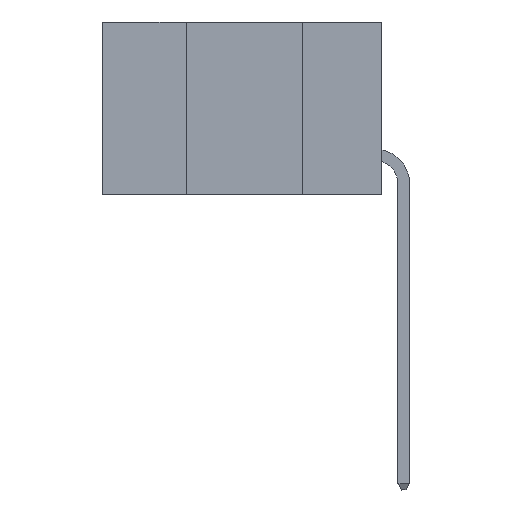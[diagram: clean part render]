
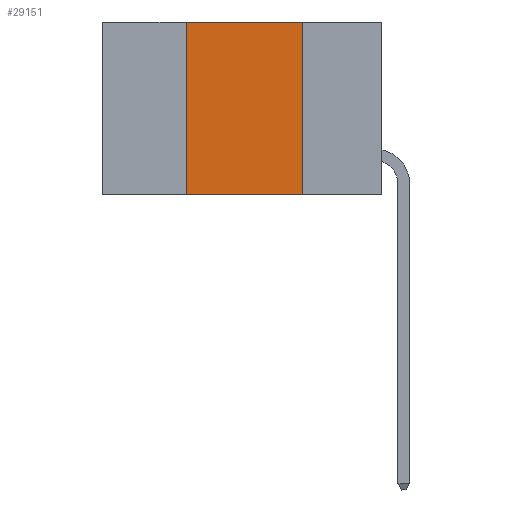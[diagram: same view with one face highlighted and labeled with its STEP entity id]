
A CAD part, left-side view. The second image highlights one B-rep face of the part: STEP entity #29151.
In plain terms, the highlighted planar face has unit normal (-1, 0, 0).
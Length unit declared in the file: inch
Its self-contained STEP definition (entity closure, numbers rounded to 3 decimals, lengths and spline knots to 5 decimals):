
#440 = ORIENTED_EDGE ( 'NONE', *, *, #24270, .F. ) ;
#1326 = CARTESIAN_POINT ( 'NONE',  ( 0., 0.17, 0. ) ) ;
#2971 = CARTESIAN_POINT ( 'NONE',  ( 0., 0.6, 0. ) ) ;
#3583 = VECTOR ( 'NONE', #29162, 39.37008 ) ;
#5345 = EDGE_CURVE ( 'NONE', #27842, #25203, #32969, .T. ) ;
#6522 = DIRECTION ( 'NONE',  ( 1., 0., 0. ) ) ;
#7519 = EDGE_CURVE ( 'NONE', #18928, #25203, #37913, .T. ) ;
#8083 = VECTOR ( 'NONE', #22757, 39.37008 ) ;
#9862 = CARTESIAN_POINT ( 'NONE',  ( 0., 0.42, -0.37 ) ) ;
#12090 = CARTESIAN_POINT ( 'NONE',  ( 0., 0.42, 0. ) ) ;
#13433 = CARTESIAN_POINT ( 'NONE',  ( 0., 0.6, 0. ) ) ;
#14147 = CARTESIAN_POINT ( 'NONE',  ( 0., 0.42, 0. ) ) ;
#14149 = DIRECTION ( 'NONE',  ( 0., 0., -1. ) ) ;
#16979 = CARTESIAN_POINT ( 'NONE',  ( 0., 0.17, 0. ) ) ;
#17227 = DIRECTION ( 'NONE',  ( 0., 0., -1. ) ) ;
#17507 = LINE ( 'NONE', #13433, #3583 ) ;
#18928 = VERTEX_POINT ( 'NONE', #9862 ) ;
#20367 = AXIS2_PLACEMENT_3D ( 'NONE', #2971, #6522, #14149 ) ;
#21437 = DIRECTION ( 'NONE',  ( 0., -1., 0. ) ) ;
#22757 = DIRECTION ( 'NONE',  ( 0., 0., 1. ) ) ;
#24270 = EDGE_CURVE ( 'NONE', #46572, #27842, #17507, .T. ) ;
#24780 = VECTOR ( 'NONE', #21437, 39.37008 ) ;
#25203 = VERTEX_POINT ( 'NONE', #30725 ) ;
#27842 = VERTEX_POINT ( 'NONE', #1326 ) ;
#29151 = ADVANCED_FACE ( 'NONE', ( #37261 ), #30114, .F. ) ;
#29162 = DIRECTION ( 'NONE',  ( 0., -1., 0. ) ) ;
#30036 = CARTESIAN_POINT ( 'NONE',  ( 0., 0.6, -0.37 ) ) ;
#30114 = PLANE ( 'NONE',  #20367 ) ;
#30371 = LINE ( 'NONE', #14147, #8083 ) ;
#30725 = CARTESIAN_POINT ( 'NONE',  ( 0., 0.17, -0.37 ) ) ;
#31342 = ORIENTED_EDGE ( 'NONE', *, *, #7519, .T. ) ;
#32969 = LINE ( 'NONE', #16979, #45984 ) ;
#37261 = FACE_OUTER_BOUND ( 'NONE', #41971, .T. ) ;
#37913 = LINE ( 'NONE', #30036, #24780 ) ;
#41512 = EDGE_CURVE ( 'NONE', #18928, #46572, #30371, .T. ) ;
#41971 = EDGE_LOOP ( 'NONE', ( #42353, #440, #48015, #31342 ) ) ;
#42353 = ORIENTED_EDGE ( 'NONE', *, *, #5345, .F. ) ;
#45984 = VECTOR ( 'NONE', #17227, 39.37008 ) ;
#46572 = VERTEX_POINT ( 'NONE', #12090 ) ;
#48015 = ORIENTED_EDGE ( 'NONE', *, *, #41512, .F. ) ;
